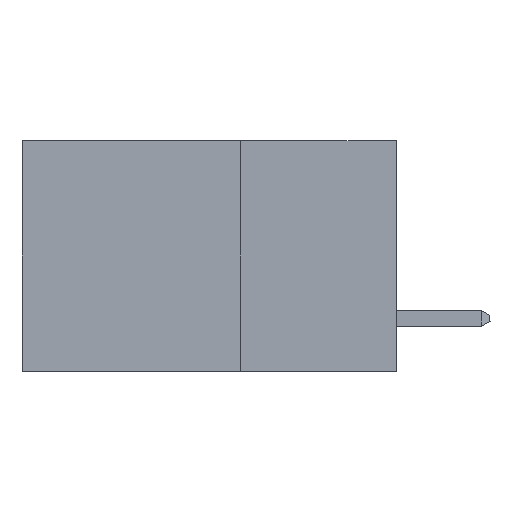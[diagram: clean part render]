
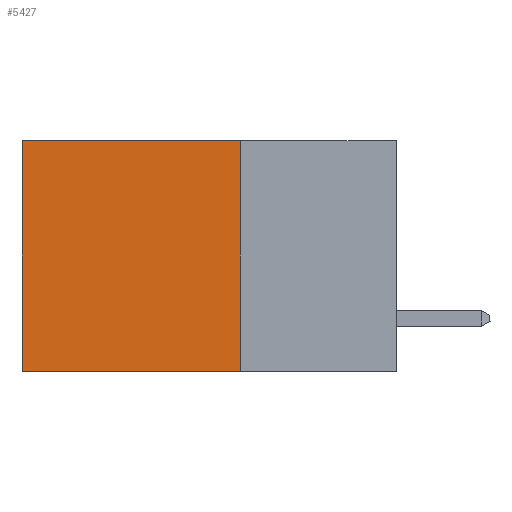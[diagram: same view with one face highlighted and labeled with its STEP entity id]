
A CAD part, left-side view. The second image highlights one B-rep face of the part: STEP entity #5427.
In plain terms, the highlighted planar face has unit normal (-1, 0, 0).
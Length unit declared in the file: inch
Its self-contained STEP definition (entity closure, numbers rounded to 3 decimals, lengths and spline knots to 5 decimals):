
#3497 = LINE ( 'NONE', #12987, #13850 ) ;
#4864 = DIRECTION ( 'NONE',  ( 0., 0., -1. ) ) ;
#4991 = DIRECTION ( 'NONE',  ( 0., 1., 0. ) ) ;
#5261 = LINE ( 'NONE', #16528, #8063 ) ;
#5427 = ADVANCED_FACE ( 'NONE', ( #16143 ), #15216, .F. ) ;
#5515 = DIRECTION ( 'NONE',  ( 0., 0., -1. ) ) ;
#7884 = EDGE_CURVE ( 'NONE', #17685, #22617, #14240, .T. ) ;
#8063 = VECTOR ( 'NONE', #4864, 39.37008 ) ;
#8077 = VERTEX_POINT ( 'NONE', #24932 ) ;
#9049 = ORIENTED_EDGE ( 'NONE', *, *, #18194, .T. ) ;
#9376 = CARTESIAN_POINT ( 'NONE',  ( 0.298, 0.25, 0. ) ) ;
#9479 = DIRECTION ( 'NONE',  ( 0., 0., -1. ) ) ;
#9788 = ORIENTED_EDGE ( 'NONE', *, *, #7884, .T. ) ;
#10450 = AXIS2_PLACEMENT_3D ( 'NONE', #9376, #17158, #5515 ) ;
#10457 = ORIENTED_EDGE ( 'NONE', *, *, #15265, .F. ) ;
#11351 = CARTESIAN_POINT ( 'NONE',  ( 0.298, 0.6, 0. ) ) ;
#12828 = CARTESIAN_POINT ( 'NONE',  ( 0.298, 0.6, 0. ) ) ;
#12987 = CARTESIAN_POINT ( 'NONE',  ( 0.298, 0.25, -0.37 ) ) ;
#13422 = CARTESIAN_POINT ( 'NONE',  ( 0.298, 0.25, 0. ) ) ;
#13782 = LINE ( 'NONE', #11351, #23985 ) ;
#13850 = VECTOR ( 'NONE', #22550, 39.37008 ) ;
#14240 = LINE ( 'NONE', #24270, #19413 ) ;
#15216 = PLANE ( 'NONE',  #10450 ) ;
#15265 = EDGE_CURVE ( 'NONE', #17685, #18405, #5261, .T. ) ;
#16143 = FACE_OUTER_BOUND ( 'NONE', #19038, .T. ) ;
#16528 = CARTESIAN_POINT ( 'NONE',  ( 0.298, 0.25, 0. ) ) ;
#16916 = EDGE_CURVE ( 'NONE', #18405, #8077, #3497, .T. ) ;
#17158 = DIRECTION ( 'NONE',  ( 1., 0., 0. ) ) ;
#17685 = VERTEX_POINT ( 'NONE', #13422 ) ;
#18194 = EDGE_CURVE ( 'NONE', #22617, #8077, #13782, .T. ) ;
#18405 = VERTEX_POINT ( 'NONE', #19749 ) ;
#19038 = EDGE_LOOP ( 'NONE', ( #9049, #24874, #10457, #9788 ) ) ;
#19413 = VECTOR ( 'NONE', #4991, 39.37008 ) ;
#19749 = CARTESIAN_POINT ( 'NONE',  ( 0.298, 0.25, -0.37 ) ) ;
#22550 = DIRECTION ( 'NONE',  ( 0., 1., 0. ) ) ;
#22617 = VERTEX_POINT ( 'NONE', #12828 ) ;
#23985 = VECTOR ( 'NONE', #9479, 39.37008 ) ;
#24270 = CARTESIAN_POINT ( 'NONE',  ( 0.298, 0.25, 0. ) ) ;
#24874 = ORIENTED_EDGE ( 'NONE', *, *, #16916, .F. ) ;
#24932 = CARTESIAN_POINT ( 'NONE',  ( 0.298, 0.6, -0.37 ) ) ;
